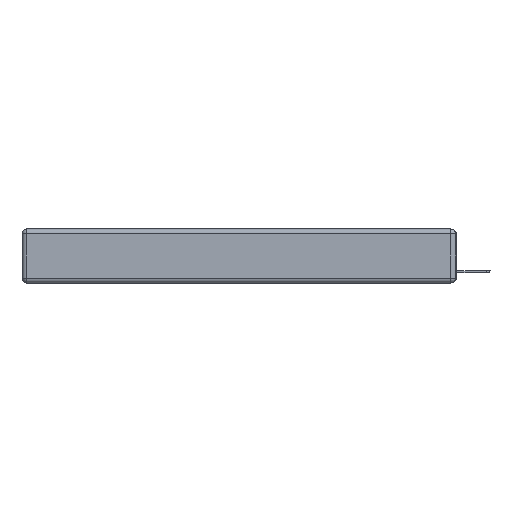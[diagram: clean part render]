
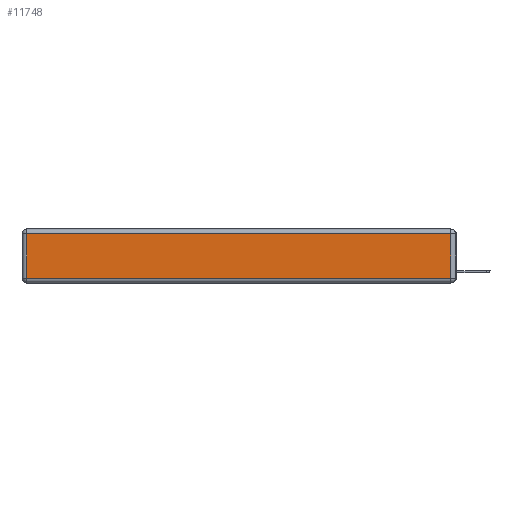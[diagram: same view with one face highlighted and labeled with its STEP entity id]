
A CAD part, left-side view. The second image highlights one B-rep face of the part: STEP entity #11748.
In plain terms, the highlighted planar face has unit normal (-1, 0, 0).
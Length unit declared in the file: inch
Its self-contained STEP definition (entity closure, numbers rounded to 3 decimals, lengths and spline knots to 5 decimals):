
#22 = CARTESIAN_POINT ( 'NONE',  ( 0., 2.72, -0.343 ) ) ;
#1358 = DIRECTION ( 'NONE',  ( 0., 0., 1. ) ) ;
#1583 = EDGE_CURVE ( 'NONE', #14208, #8328, #7106, .T. ) ;
#1927 = VECTOR ( 'NONE', #13703, 39.37008 ) ;
#2175 = CARTESIAN_POINT ( 'NONE',  ( 0., 0., -0.313 ) ) ;
#2757 = DIRECTION ( 'NONE',  ( -1., 0., 0. ) ) ;
#2991 = CARTESIAN_POINT ( 'NONE',  ( 0., 2.72, -0.03 ) ) ;
#3288 = LINE ( 'NONE', #16645, #1927 ) ;
#3463 = EDGE_CURVE ( 'NONE', #8328, #18032, #6585, .T. ) ;
#3501 = DIRECTION ( 'NONE',  ( 0., -1., 0. ) ) ;
#4311 = LINE ( 'NONE', #22, #18255 ) ;
#4367 = VECTOR ( 'NONE', #3501, 39.37008 ) ;
#4817 = CARTESIAN_POINT ( 'NONE',  ( 0., 0.03, -0.343 ) ) ;
#6585 = LINE ( 'NONE', #4817, #10235 ) ;
#7092 = PLANE ( 'NONE',  #10468 ) ;
#7106 = LINE ( 'NONE', #2175, #4367 ) ;
#8328 = VERTEX_POINT ( 'NONE', #15819 ) ;
#8585 = EDGE_LOOP ( 'NONE', ( #14692, #11333, #16540, #11513 ) ) ;
#8889 = DIRECTION ( 'NONE',  ( 0., 0., -1. ) ) ;
#10235 = VECTOR ( 'NONE', #17871, 39.37008 ) ;
#10468 = AXIS2_PLACEMENT_3D ( 'NONE', #17293, #2757, #1358 ) ;
#11333 = ORIENTED_EDGE ( 'NONE', *, *, #3463, .T. ) ;
#11513 = ORIENTED_EDGE ( 'NONE', *, *, #13993, .T. ) ;
#11748 = ADVANCED_FACE ( 'NONE', ( #14536 ), #7092, .T. ) ;
#12192 = CARTESIAN_POINT ( 'NONE',  ( 0., 0.03, -0.03 ) ) ;
#12471 = CARTESIAN_POINT ( 'NONE',  ( 0., 2.72, -0.313 ) ) ;
#13703 = DIRECTION ( 'NONE',  ( 0., 1., 0. ) ) ;
#13993 = EDGE_CURVE ( 'NONE', #14512, #14208, #4311, .T. ) ;
#14208 = VERTEX_POINT ( 'NONE', #12471 ) ;
#14512 = VERTEX_POINT ( 'NONE', #2991 ) ;
#14536 = FACE_OUTER_BOUND ( 'NONE', #8585, .T. ) ;
#14692 = ORIENTED_EDGE ( 'NONE', *, *, #1583, .T. ) ;
#15819 = CARTESIAN_POINT ( 'NONE',  ( 0., 0.03, -0.313 ) ) ;
#16540 = ORIENTED_EDGE ( 'NONE', *, *, #16795, .T. ) ;
#16645 = CARTESIAN_POINT ( 'NONE',  ( 0., 2.75, -0.03 ) ) ;
#16795 = EDGE_CURVE ( 'NONE', #18032, #14512, #3288, .T. ) ;
#17293 = CARTESIAN_POINT ( 'NONE',  ( 0., 0., -0.343 ) ) ;
#17871 = DIRECTION ( 'NONE',  ( 0., 0., 1. ) ) ;
#18032 = VERTEX_POINT ( 'NONE', #12192 ) ;
#18255 = VECTOR ( 'NONE', #8889, 39.37008 ) ;
